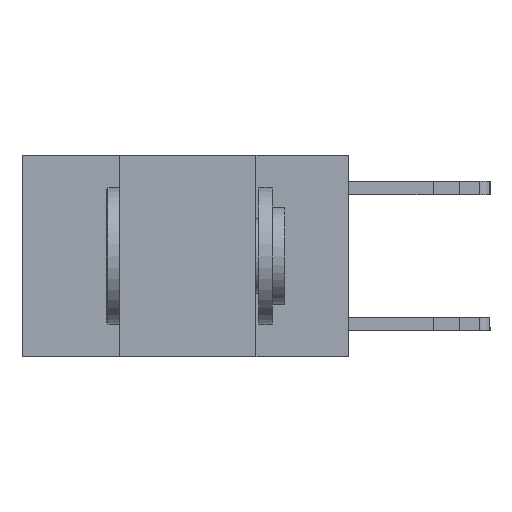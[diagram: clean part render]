
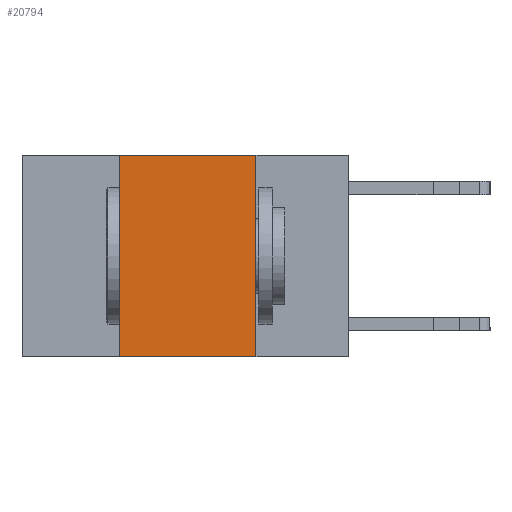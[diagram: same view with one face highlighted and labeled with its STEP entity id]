
A CAD part, left-side view. The second image highlights one B-rep face of the part: STEP entity #20794.
In plain terms, the highlighted planar face has unit normal (-1, 0, 0).
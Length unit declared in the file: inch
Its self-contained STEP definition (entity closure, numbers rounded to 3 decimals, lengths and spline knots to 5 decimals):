
#937 = LINE ( 'NONE', #13758, #18985 ) ;
#1031 = FACE_OUTER_BOUND ( 'NONE', #25525, .T. ) ;
#1159 = CARTESIAN_POINT ( 'NONE',  ( 0., 0.6, 0. ) ) ;
#2653 = CARTESIAN_POINT ( 'NONE',  ( 0., 0.17, -0.37 ) ) ;
#3452 = DIRECTION ( 'NONE',  ( 0., 0., -1. ) ) ;
#3622 = CARTESIAN_POINT ( 'NONE',  ( 0., 0.6, -0.37 ) ) ;
#4015 = LINE ( 'NONE', #3622, #23227 ) ;
#4063 = VERTEX_POINT ( 'NONE', #13335 ) ;
#4819 = LINE ( 'NONE', #23414, #7012 ) ;
#4954 = DIRECTION ( 'NONE',  ( 0., 0., -1. ) ) ;
#5424 = VECTOR ( 'NONE', #21946, 39.37008 ) ;
#7012 = VECTOR ( 'NONE', #4954, 39.37008 ) ;
#11267 = EDGE_CURVE ( 'NONE', #20174, #20705, #4819, .T. ) ;
#11457 = CARTESIAN_POINT ( 'NONE',  ( 0., 0.6, 0. ) ) ;
#11469 = ORIENTED_EDGE ( 'NONE', *, *, #11267, .F. ) ;
#11815 = VERTEX_POINT ( 'NONE', #25994 ) ;
#12300 = AXIS2_PLACEMENT_3D ( 'NONE', #1159, #21525, #3452 ) ;
#13335 = CARTESIAN_POINT ( 'NONE',  ( 0., 0.42, -0.37 ) ) ;
#13513 = EDGE_CURVE ( 'NONE', #4063, #11815, #937, .T. ) ;
#13758 = CARTESIAN_POINT ( 'NONE',  ( 0., 0.42, 0. ) ) ;
#14468 = ORIENTED_EDGE ( 'NONE', *, *, #13513, .F. ) ;
#16613 = ORIENTED_EDGE ( 'NONE', *, *, #26123, .T. ) ;
#18330 = DIRECTION ( 'NONE',  ( 0., -1., 0. ) ) ;
#18985 = VECTOR ( 'NONE', #25588, 39.37008 ) ;
#19656 = PLANE ( 'NONE',  #12300 ) ;
#20174 = VERTEX_POINT ( 'NONE', #23037 ) ;
#20705 = VERTEX_POINT ( 'NONE', #2653 ) ;
#20794 = ADVANCED_FACE ( 'NONE', ( #1031 ), #19656, .F. ) ;
#21525 = DIRECTION ( 'NONE',  ( 1., 0., 0. ) ) ;
#21700 = LINE ( 'NONE', #11457, #5424 ) ;
#21857 = EDGE_CURVE ( 'NONE', #11815, #20174, #21700, .T. ) ;
#21946 = DIRECTION ( 'NONE',  ( 0., -1., 0. ) ) ;
#23037 = CARTESIAN_POINT ( 'NONE',  ( 0., 0.17, 0. ) ) ;
#23227 = VECTOR ( 'NONE', #18330, 39.37008 ) ;
#23414 = CARTESIAN_POINT ( 'NONE',  ( 0., 0.17, 0. ) ) ;
#24333 = ORIENTED_EDGE ( 'NONE', *, *, #21857, .F. ) ;
#25525 = EDGE_LOOP ( 'NONE', ( #11469, #24333, #14468, #16613 ) ) ;
#25588 = DIRECTION ( 'NONE',  ( 0., 0., 1. ) ) ;
#25994 = CARTESIAN_POINT ( 'NONE',  ( 0., 0.42, 0. ) ) ;
#26123 = EDGE_CURVE ( 'NONE', #4063, #20705, #4015, .T. ) ;
